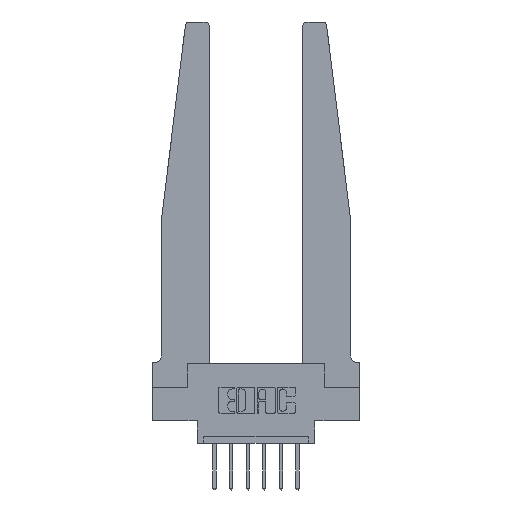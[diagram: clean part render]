
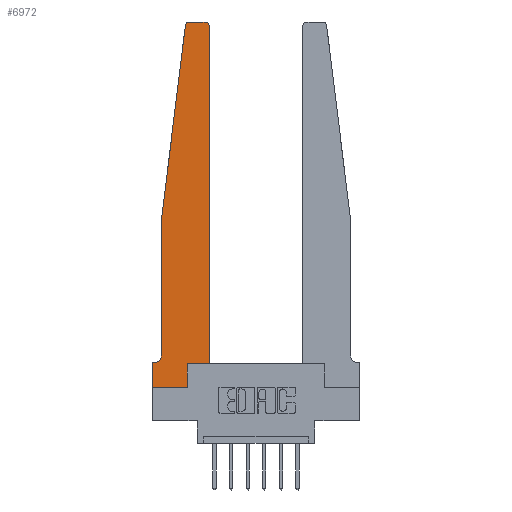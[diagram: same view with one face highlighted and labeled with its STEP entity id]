
A CAD part, top view. The second image highlights one B-rep face of the part: STEP entity #6972.
In plain terms, the highlighted planar face has unit normal (0, 0, 1).
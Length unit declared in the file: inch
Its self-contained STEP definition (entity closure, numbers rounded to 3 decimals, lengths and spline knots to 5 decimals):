
#7 = DIRECTION ( 'NONE',  ( 0., -1., 0. ) ) ;
#64 = LINE ( 'NONE', #5846, #5568 ) ;
#119 = ORIENTED_EDGE ( 'NONE', *, *, #1901, .T. ) ;
#210 = EDGE_CURVE ( 'NONE', #11443, #13827, #9661, .T. ) ;
#236 = CARTESIAN_POINT ( 'NONE',  ( 0.2605, 0., 0.37 ) ) ;
#242 = VERTEX_POINT ( 'NONE', #956 ) ;
#469 = EDGE_CURVE ( 'NONE', #7011, #2302, #12398, .T. ) ;
#956 = CARTESIAN_POINT ( 'NONE',  ( 0.24675, 2.72367, 0.37 ) ) ;
#1003 = AXIS2_PLACEMENT_3D ( 'NONE', #2648, #7972, #5788 ) ;
#1192 = ORIENTED_EDGE ( 'NONE', *, *, #11241, .T. ) ;
#1207 = CARTESIAN_POINT ( 'NONE',  ( 0.065, 1.25, 0.37 ) ) ;
#1213 = EDGE_CURVE ( 'NONE', #2302, #3957, #64, .T. ) ;
#1272 = VECTOR ( 'NONE', #7, 39.37008 ) ;
#1284 = VECTOR ( 'NONE', #7218, 39.37008 ) ;
#1648 = ORIENTED_EDGE ( 'NONE', *, *, #12997, .T. ) ;
#1762 = ORIENTED_EDGE ( 'NONE', *, *, #2235, .T. ) ;
#1901 = EDGE_CURVE ( 'NONE', #6122, #10834, #6297, .T. ) ;
#2184 = CARTESIAN_POINT ( 'NONE',  ( 0.25, 2.75, 0.37 ) ) ;
#2235 = EDGE_CURVE ( 'NONE', #2883, #5064, #8544, .T. ) ;
#2302 = VERTEX_POINT ( 'NONE', #2484 ) ;
#2484 = CARTESIAN_POINT ( 'NONE',  ( 0.2605, 0.18, 0.37 ) ) ;
#2634 = ORIENTED_EDGE ( 'NONE', *, *, #5404, .T. ) ;
#2648 = CARTESIAN_POINT ( 'NONE',  ( 0.27653, 2.72, 0.37 ) ) ;
#2806 = AXIS2_PLACEMENT_3D ( 'NONE', #12836, #3330, #5471 ) ;
#2810 = CARTESIAN_POINT ( 'NONE',  ( 0.2605, 0.18, 0.37 ) ) ;
#2883 = VERTEX_POINT ( 'NONE', #11928 ) ;
#2897 = DIRECTION ( 'NONE',  ( -1., 0., 0. ) ) ;
#3326 = CIRCLE ( 'NONE', #7566, 0.05 ) ;
#3330 = DIRECTION ( 'NONE',  ( 0., 0., 1. ) ) ;
#3366 = LINE ( 'NONE', #7635, #12022 ) ;
#3407 = DIRECTION ( 'NONE',  ( -1., 0., 0. ) ) ;
#3592 = CARTESIAN_POINT ( 'NONE',  ( 0.425, 0.18, 0.37 ) ) ;
#3957 = VERTEX_POINT ( 'NONE', #12351 ) ;
#4228 = EDGE_CURVE ( 'NONE', #10085, #11443, #4961, .T. ) ;
#4619 = VECTOR ( 'NONE', #5870, 39.37008 ) ;
#4961 = LINE ( 'NONE', #9212, #10212 ) ;
#5064 = VERTEX_POINT ( 'NONE', #11595 ) ;
#5270 = CARTESIAN_POINT ( 'NONE',  ( 0.395, 2.72, 0.37 ) ) ;
#5404 = EDGE_CURVE ( 'NONE', #242, #6122, #7964, .T. ) ;
#5471 = DIRECTION ( 'NONE',  ( 1., 0., 0. ) ) ;
#5568 = VECTOR ( 'NONE', #13347, 39.37008 ) ;
#5788 = DIRECTION ( 'NONE',  ( 1., 0., 0. ) ) ;
#5846 = CARTESIAN_POINT ( 'NONE',  ( 0.425, 0.18, 0.37 ) ) ;
#5870 = DIRECTION ( 'NONE',  ( 0., 1., 0. ) ) ;
#5889 = EDGE_LOOP ( 'NONE', ( #1762, #10413, #2634, #119, #6914, #13145, #10199, #1192, #10407, #13690, #11779, #1648 ) ) ;
#6122 = VERTEX_POINT ( 'NONE', #11665 ) ;
#6297 = LINE ( 'NONE', #7289, #9060 ) ;
#6337 = CARTESIAN_POINT ( 'NONE',  ( 0.425, 2.72, 0.37 ) ) ;
#6386 = FACE_OUTER_BOUND ( 'NONE', #5889, .T. ) ;
#6581 = CARTESIAN_POINT ( 'NONE',  ( 0., 0., 0.37 ) ) ;
#6868 = VECTOR ( 'NONE', #3407, 39.37008 ) ;
#6873 = LINE ( 'NONE', #3592, #4619 ) ;
#6914 = ORIENTED_EDGE ( 'NONE', *, *, #10953, .T. ) ;
#6972 = ADVANCED_FACE ( 'NONE', ( #6386 ), #10658, .T. ) ;
#7011 = VERTEX_POINT ( 'NONE', #236 ) ;
#7218 = DIRECTION ( 'NONE',  ( 0., 1., 0. ) ) ;
#7289 = CARTESIAN_POINT ( 'NONE',  ( 0.065, 1.25, 0.37 ) ) ;
#7421 = DIRECTION ( 'NONE',  ( 0., -1., 0. ) ) ;
#7453 = DIRECTION ( 'NONE',  ( 1., 0., 0. ) ) ;
#7550 = VECTOR ( 'NONE', #13218, 39.37008 ) ;
#7566 = AXIS2_PLACEMENT_3D ( 'NONE', #10305, #13516, #2897 ) ;
#7635 = CARTESIAN_POINT ( 'NONE',  ( 0., 0., 0.37 ) ) ;
#7654 = AXIS2_PLACEMENT_3D ( 'NONE', #5270, #10583, #7453 ) ;
#7855 = CARTESIAN_POINT ( 'NONE',  ( 0., 0., 0.37 ) ) ;
#7964 = LINE ( 'NONE', #1207, #7550 ) ;
#7972 = DIRECTION ( 'NONE',  ( 0., 0., 1. ) ) ;
#7975 = DIRECTION ( 'NONE',  ( 1., 0., 0. ) ) ;
#8370 = EDGE_CURVE ( 'NONE', #3957, #10001, #6873, .T. ) ;
#8544 = LINE ( 'NONE', #2184, #6868 ) ;
#8751 = EDGE_CURVE ( 'NONE', #5064, #242, #11342, .T. ) ;
#9060 = VECTOR ( 'NONE', #7421, 39.37008 ) ;
#9212 = CARTESIAN_POINT ( 'NONE',  ( 0.065, 0.1875, 0.37 ) ) ;
#9619 = DIRECTION ( 'NONE',  ( -1., 0., 0. ) ) ;
#9661 = LINE ( 'NONE', #6581, #1272 ) ;
#10001 = VERTEX_POINT ( 'NONE', #6337 ) ;
#10085 = VERTEX_POINT ( 'NONE', #12232 ) ;
#10135 = CARTESIAN_POINT ( 'NONE',  ( 0., 0.1875, 0.37 ) ) ;
#10199 = ORIENTED_EDGE ( 'NONE', *, *, #210, .T. ) ;
#10212 = VECTOR ( 'NONE', #9619, 39.37008 ) ;
#10305 = CARTESIAN_POINT ( 'NONE',  ( 0.015, 0.2375, 0.37 ) ) ;
#10407 = ORIENTED_EDGE ( 'NONE', *, *, #469, .T. ) ;
#10413 = ORIENTED_EDGE ( 'NONE', *, *, #8751, .T. ) ;
#10583 = DIRECTION ( 'NONE',  ( 0., 0., 1. ) ) ;
#10658 = PLANE ( 'NONE',  #2806 ) ;
#10834 = VERTEX_POINT ( 'NONE', #13240 ) ;
#10953 = EDGE_CURVE ( 'NONE', #10834, #10085, #3326, .T. ) ;
#11241 = EDGE_CURVE ( 'NONE', #13827, #7011, #3366, .T. ) ;
#11342 = CIRCLE ( 'NONE', #1003, 0.03 ) ;
#11443 = VERTEX_POINT ( 'NONE', #10135 ) ;
#11595 = CARTESIAN_POINT ( 'NONE',  ( 0.27653, 2.75, 0.37 ) ) ;
#11665 = CARTESIAN_POINT ( 'NONE',  ( 0.065, 1.25, 0.37 ) ) ;
#11779 = ORIENTED_EDGE ( 'NONE', *, *, #8370, .T. ) ;
#11928 = CARTESIAN_POINT ( 'NONE',  ( 0.395, 2.75, 0.37 ) ) ;
#12022 = VECTOR ( 'NONE', #7975, 39.37008 ) ;
#12232 = CARTESIAN_POINT ( 'NONE',  ( 0.015, 0.1875, 0.37 ) ) ;
#12351 = CARTESIAN_POINT ( 'NONE',  ( 0.425, 0.18, 0.37 ) ) ;
#12398 = LINE ( 'NONE', #2810, #1284 ) ;
#12836 = CARTESIAN_POINT ( 'NONE',  ( 0., 0.1875, 0.37 ) ) ;
#12997 = EDGE_CURVE ( 'NONE', #10001, #2883, #13675, .T. ) ;
#13145 = ORIENTED_EDGE ( 'NONE', *, *, #4228, .T. ) ;
#13218 = DIRECTION ( 'NONE',  ( -0.122, -0.992, 0. ) ) ;
#13240 = CARTESIAN_POINT ( 'NONE',  ( 0.065, 0.2375, 0.37 ) ) ;
#13347 = DIRECTION ( 'NONE',  ( 1., 0., 0. ) ) ;
#13516 = DIRECTION ( 'NONE',  ( 0., 0., -1. ) ) ;
#13675 = CIRCLE ( 'NONE', #7654, 0.03 ) ;
#13690 = ORIENTED_EDGE ( 'NONE', *, *, #1213, .T. ) ;
#13827 = VERTEX_POINT ( 'NONE', #7855 ) ;
